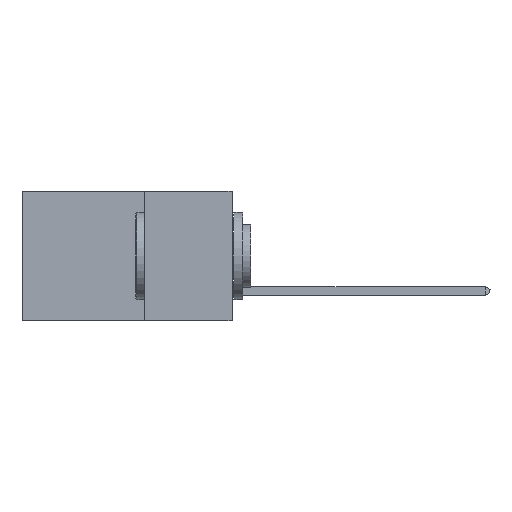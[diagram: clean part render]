
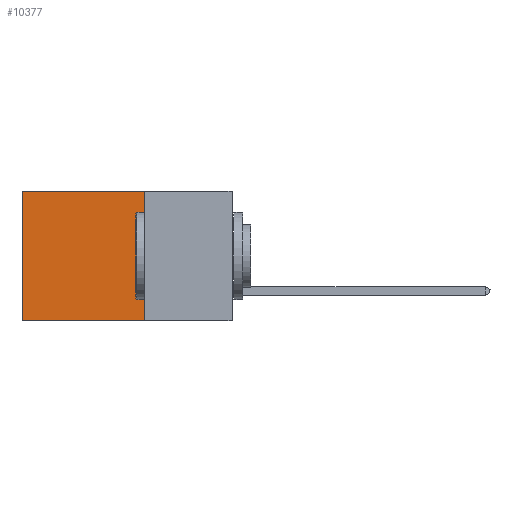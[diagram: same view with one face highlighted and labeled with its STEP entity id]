
A CAD part, left-side view. The second image highlights one B-rep face of the part: STEP entity #10377.
In plain terms, the highlighted planar face has unit normal (-1, 0, 0).
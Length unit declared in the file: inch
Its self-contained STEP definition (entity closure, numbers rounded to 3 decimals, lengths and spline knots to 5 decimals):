
#876 = EDGE_CURVE ( 'NONE', #10233, #9009, #7191, .T. ) ;
#1097 = CARTESIAN_POINT ( 'NONE',  ( 0.2875, 0.25, -0.37 ) ) ;
#1983 = FACE_OUTER_BOUND ( 'NONE', #3322, .T. ) ;
#2086 = ORIENTED_EDGE ( 'NONE', *, *, #14032, .T. ) ;
#2447 = CARTESIAN_POINT ( 'NONE',  ( 0.2875, 0.25, -0.37 ) ) ;
#3097 = LINE ( 'NONE', #5884, #16706 ) ;
#3174 = CARTESIAN_POINT ( 'NONE',  ( 0.2875, 0.6, 0. ) ) ;
#3234 = LINE ( 'NONE', #2447, #17486 ) ;
#3322 = EDGE_LOOP ( 'NONE', ( #2086, #5860, #6092, #6921 ) ) ;
#5174 = LINE ( 'NONE', #8219, #15325 ) ;
#5690 = CARTESIAN_POINT ( 'NONE',  ( 0.2875, 0.25, 0. ) ) ;
#5817 = DIRECTION ( 'NONE',  ( 1., 0., 0. ) ) ;
#5860 = ORIENTED_EDGE ( 'NONE', *, *, #13635, .F. ) ;
#5884 = CARTESIAN_POINT ( 'NONE',  ( 0.2875, 0.25, 0. ) ) ;
#6092 = ORIENTED_EDGE ( 'NONE', *, *, #876, .F. ) ;
#6216 = CARTESIAN_POINT ( 'NONE',  ( 0.2875, 0.25, 0. ) ) ;
#6271 = VERTEX_POINT ( 'NONE', #16636 ) ;
#6528 = AXIS2_PLACEMENT_3D ( 'NONE', #8492, #5817, #16895 ) ;
#6727 = DIRECTION ( 'NONE',  ( 0., 1., 0. ) ) ;
#6921 = ORIENTED_EDGE ( 'NONE', *, *, #9836, .T. ) ;
#7191 = LINE ( 'NONE', #6216, #9106 ) ;
#8219 = CARTESIAN_POINT ( 'NONE',  ( 0.2875, 0.6, 0. ) ) ;
#8275 = DIRECTION ( 'NONE',  ( 0., 0., -1. ) ) ;
#8492 = CARTESIAN_POINT ( 'NONE',  ( 0.2875, 0.25, 0. ) ) ;
#9009 = VERTEX_POINT ( 'NONE', #1097 ) ;
#9106 = VECTOR ( 'NONE', #15866, 39.37008 ) ;
#9836 = EDGE_CURVE ( 'NONE', #10233, #10744, #3097, .T. ) ;
#9886 = DIRECTION ( 'NONE',  ( 0., 1., 0. ) ) ;
#10233 = VERTEX_POINT ( 'NONE', #5690 ) ;
#10377 = ADVANCED_FACE ( 'NONE', ( #1983 ), #13936, .F. ) ;
#10744 = VERTEX_POINT ( 'NONE', #3174 ) ;
#13635 = EDGE_CURVE ( 'NONE', #9009, #6271, #3234, .T. ) ;
#13936 = PLANE ( 'NONE',  #6528 ) ;
#14032 = EDGE_CURVE ( 'NONE', #10744, #6271, #5174, .T. ) ;
#15325 = VECTOR ( 'NONE', #8275, 39.37008 ) ;
#15866 = DIRECTION ( 'NONE',  ( 0., 0., -1. ) ) ;
#16636 = CARTESIAN_POINT ( 'NONE',  ( 0.2875, 0.6, -0.37 ) ) ;
#16706 = VECTOR ( 'NONE', #9886, 39.37008 ) ;
#16895 = DIRECTION ( 'NONE',  ( 0., 0., -1. ) ) ;
#17486 = VECTOR ( 'NONE', #6727, 39.37008 ) ;
